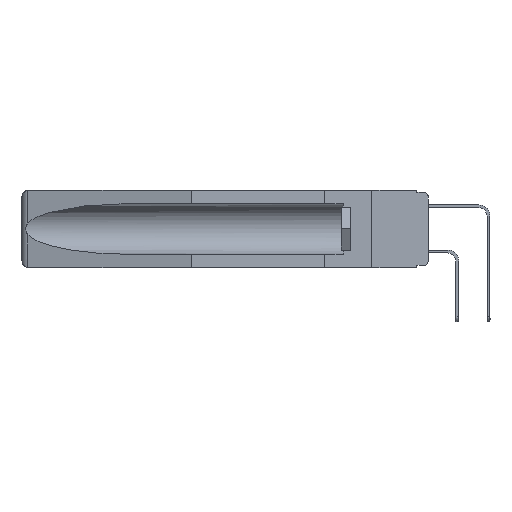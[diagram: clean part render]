
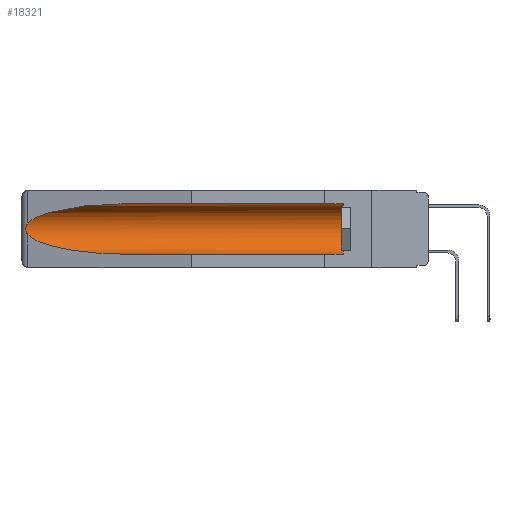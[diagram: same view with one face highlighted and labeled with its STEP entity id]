
A CAD part, left-side view. The second image highlights one B-rep face of the part: STEP entity #18321.
In plain terms, the highlighted cylindrical face has radius 2.857 mm (diameter 5.715 mm), a partial arc.
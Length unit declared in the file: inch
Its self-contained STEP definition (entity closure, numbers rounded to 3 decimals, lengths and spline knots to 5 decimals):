
#341 = CARTESIAN_POINT ( 'NONE',  ( 0.155, -0.30754, -0.284 ) ) ;
#550 = CARTESIAN_POINT ( 'NONE',  ( 0.155, -0.30754, -0.059 ) ) ;
#628 = DIRECTION ( 'NONE',  ( 0., 1., 0. ) ) ;
#2726 = CARTESIAN_POINT ( 'NONE',  ( 0.155, 0.126, -0.059 ) ) ;
#2933 = ORIENTED_EDGE ( 'NONE', *, *, #18202, .T. ) ;
#3406 = CARTESIAN_POINT ( 'NONE',  ( 0.155, 1.07973, -0.284 ) ) ;
#3980 = CARTESIAN_POINT ( 'NONE',  ( 0.26597, 1.5296, -0.19026 ) ) ;
#4062 = CARTESIAN_POINT ( 'NONE',  ( 0.26537, 1.52718, -0.14972 ) ) ;
#4278 = CARTESIAN_POINT ( 'NONE',  ( 0.26654, 1.53092, -0.15636 ) ) ;
#4355 = CIRCLE ( 'NONE', #4459, 0.1125 ) ;
#4459 = AXIS2_PLACEMENT_3D ( 'NONE', #19966, #5448, #8785 ) ;
#4581 = VECTOR ( 'NONE', #20121, 39.37008 ) ;
#5056 = CARTESIAN_POINT ( 'NONE',  ( 0.21114, 1.30732, -0.059 ) ) ;
#5317 = CARTESIAN_POINT ( 'NONE',  ( 0.26537, 1.52718, -0.14972 ) ) ;
#5433 =( BOUNDED_CURVE ( )  B_SPLINE_CURVE ( 3, ( #14082, #16071, #14408, #3406 ),
 .UNSPECIFIED., .F., .F. ) 
 B_SPLINE_CURVE_WITH_KNOTS ( ( 4, 4 ),
 ( 0.1948, 1.5708 ),
 .UNSPECIFIED. ) 
 CURVE ( )  GEOMETRIC_REPRESENTATION_ITEM ( )  RATIONAL_B_SPLINE_CURVE ( ( 1., 0.848, 0.848, 1. ) ) 
 REPRESENTATION_ITEM ( '' )  );
#5440 = CARTESIAN_POINT ( 'NONE',  ( 0.26537, 1.52718, -0.19328 ) ) ;
#5448 = DIRECTION ( 'NONE',  ( 0., -1., 0. ) ) ;
#5891 = ORIENTED_EDGE ( 'NONE', *, *, #23318, .T. ) ;
#6335 = VECTOR ( 'NONE', #628, 39.37008 ) ;
#6864 = EDGE_LOOP ( 'NONE', ( #2933, #5891, #23345, #23529, #12344, #7480 ) ) ;
#7448 = DIRECTION ( 'NONE',  ( 0., 1., 0. ) ) ;
#7480 = ORIENTED_EDGE ( 'NONE', *, *, #17907, .T. ) ;
#7754 = LINE ( 'NONE', #550, #6335 ) ;
#8785 = DIRECTION ( 'NONE',  ( 0., 0., 1. ) ) ;
#9142 = VERTEX_POINT ( 'NONE', #5317 ) ;
#9778 = CARTESIAN_POINT ( 'NONE',  ( 0.2673, 1.5327, -0.16383 ) ) ;
#10365 = B_SPLINE_CURVE_WITH_KNOTS ( 'NONE', 3,
 ( #4062, #22347, #4278, #9778, #22573, #13068, #11581, #14922, #3980, #18570 ),
 .UNSPECIFIED., .F., .F.,
 ( 4, 2, 2, 2, 4 ),
 ( 0., 0.00029, 0.00058, 0.00087, 0.00117 ),
 .UNSPECIFIED. ) ;
#11581 = CARTESIAN_POINT ( 'NONE',  ( 0.2673, 1.53269, -0.17917 ) ) ;
#11849 = EDGE_CURVE ( 'NONE', #18861, #16014, #5433, .T. ) ;
#12187 = CARTESIAN_POINT ( 'NONE',  ( 0.26537, 1.52718, -0.14972 ) ) ;
#12344 = ORIENTED_EDGE ( 'NONE', *, *, #16995, .T. ) ;
#12520 = CARTESIAN_POINT ( 'NONE',  ( 0.155, 1.07973, -0.059 ) ) ;
#12856 = FACE_OUTER_BOUND ( 'NONE', #6864, .T. ) ;
#12942 = CARTESIAN_POINT ( 'NONE',  ( 0.155, -0.30754, -0.1715 ) ) ;
#13068 = CARTESIAN_POINT ( 'NONE',  ( 0.2675, 1.53308, -0.17534 ) ) ;
#13928 = CARTESIAN_POINT ( 'NONE',  ( 0.155, 1.07973, -0.284 ) ) ;
#14082 = CARTESIAN_POINT ( 'NONE',  ( 0.26537, 1.52718, -0.19328 ) ) ;
#14298 = CYLINDRICAL_SURFACE ( 'NONE', #22545, 0.1125 ) ;
#14408 = CARTESIAN_POINT ( 'NONE',  ( 0.21114, 1.30732, -0.284 ) ) ;
#14922 = CARTESIAN_POINT ( 'NONE',  ( 0.26655, 1.53094, -0.18657 ) ) ;
#16014 = VERTEX_POINT ( 'NONE', #13928 ) ;
#16071 = CARTESIAN_POINT ( 'NONE',  ( 0.25451, 1.48313, -0.24835 ) ) ;
#16995 = EDGE_CURVE ( 'NONE', #19098, #22157, #4355, .T. ) ;
#17374 = LINE ( 'NONE', #341, #4581 ) ;
#17884 = CARTESIAN_POINT ( 'NONE',  ( 0.25451, 1.48313, -0.09465 ) ) ;
#17907 = EDGE_CURVE ( 'NONE', #22157, #18177, #7754, .T. ) ;
#18177 = VERTEX_POINT ( 'NONE', #12520 ) ;
#18202 = EDGE_CURVE ( 'NONE', #18177, #9142, #23437, .T. ) ;
#18321 = ADVANCED_FACE ( 'NONE', ( #12856 ), #14298, .F. ) ;
#18350 = CARTESIAN_POINT ( 'NONE',  ( 0.155, 0.126, -0.284 ) ) ;
#18570 = CARTESIAN_POINT ( 'NONE',  ( 0.26537, 1.52718, -0.19328 ) ) ;
#18861 = VERTEX_POINT ( 'NONE', #5440 ) ;
#18962 = EDGE_CURVE ( 'NONE', #19098, #16014, #17374, .T. ) ;
#19098 = VERTEX_POINT ( 'NONE', #18350 ) ;
#19966 = CARTESIAN_POINT ( 'NONE',  ( 0.155, 0.126, -0.1715 ) ) ;
#20121 = DIRECTION ( 'NONE',  ( 0., 1., 0. ) ) ;
#21838 = DIRECTION ( 'NONE',  ( 0., 0., 1. ) ) ;
#22157 = VERTEX_POINT ( 'NONE', #2726 ) ;
#22347 = CARTESIAN_POINT ( 'NONE',  ( 0.26597, 1.52961, -0.15275 ) ) ;
#22545 = AXIS2_PLACEMENT_3D ( 'NONE', #12942, #7448, #21838 ) ;
#22573 = CARTESIAN_POINT ( 'NONE',  ( 0.2675, 1.53308, -0.16763 ) ) ;
#23185 = CARTESIAN_POINT ( 'NONE',  ( 0.155, 1.07973, -0.059 ) ) ;
#23318 = EDGE_CURVE ( 'NONE', #9142, #18861, #10365, .T. ) ;
#23345 = ORIENTED_EDGE ( 'NONE', *, *, #11849, .T. ) ;
#23437 =( BOUNDED_CURVE ( )  B_SPLINE_CURVE ( 3, ( #23185, #5056, #17884, #12187 ),
 .UNSPECIFIED., .F., .F. ) 
 B_SPLINE_CURVE_WITH_KNOTS ( ( 4, 4 ),
 ( 4.71239, 6.08839 ),
 .UNSPECIFIED. ) 
 CURVE ( )  GEOMETRIC_REPRESENTATION_ITEM ( )  RATIONAL_B_SPLINE_CURVE ( ( 1., 0.848, 0.848, 1. ) ) 
 REPRESENTATION_ITEM ( '' )  );
#23529 = ORIENTED_EDGE ( 'NONE', *, *, #18962, .F. ) ;
